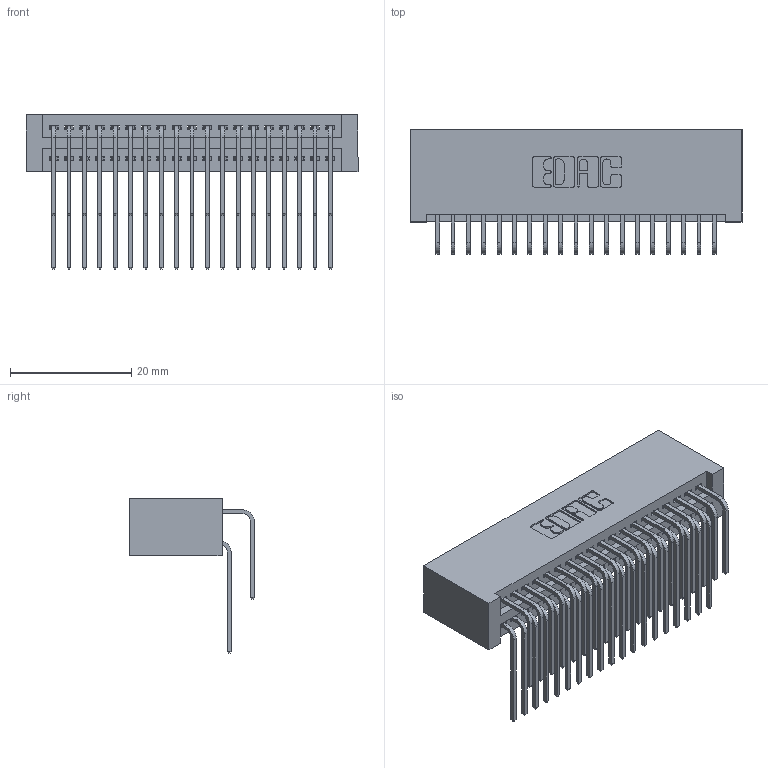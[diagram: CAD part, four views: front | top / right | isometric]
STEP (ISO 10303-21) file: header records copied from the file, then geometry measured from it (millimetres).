
FILE_DESCRIPTION (( 'STEP AP203' ), '1' );
FILE_NAME ('395-038-559-201.STEP', '2019-10-18T04:32:59', ( '' ), ( '' ), 'SwSTEP 2.0', 'SolidWorks 2016', '' );
FILE_SCHEMA (( 'CONFIG_CONTROL_DESIGN' ));
Length unit declared in the file: inch
Products named in the file (4): 345-292-001_559 Tail - 2; 395-038-559-201; 345 Part_No Mounting Lugs; 345-292-001_558 559 Tail - 1
Assembly tree (39 placements, depth 2):
  395-038-559-201
    345 Part_No Mounting Lugs
    345-292-001_558 559 Tail - 1  x19
    345-292-001_559 Tail - 2  x19
Bounding box: 54.86 x 20.56 x 25.53 mm (x, y, z)
Volume: 5951.2 mm3; surface area: 9685.4 mm2
Topology: 39 solids, 39 shells, 2094 faces, 6207 edges, 4086 vertices
Faces by surface type: plane 1406, cylinder 688
Entity records: 19379 total; most frequent: CARTESIAN_POINT 3315, ORIENTED_EDGE 3198, DIRECTION 2919, EDGE_CURVE 1599, LINE 1359, VECTOR 1359, VERTEX_POINT 1062, AXIS2_PLACEMENT_3D 780
